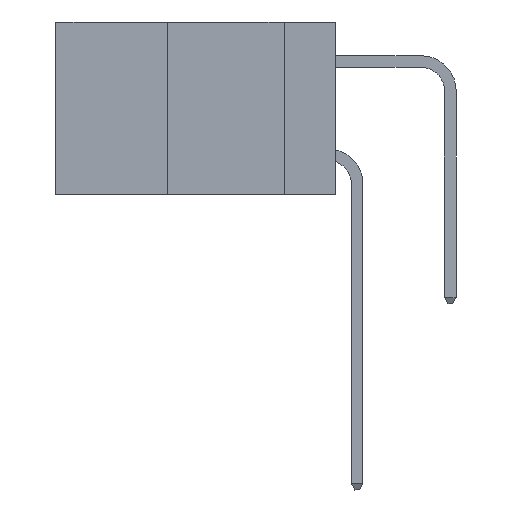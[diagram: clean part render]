
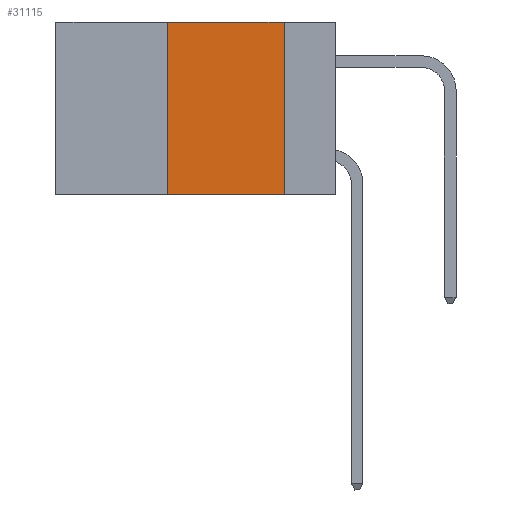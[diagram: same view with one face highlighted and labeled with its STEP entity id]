
A CAD part, left-side view. The second image highlights one B-rep face of the part: STEP entity #31115.
In plain terms, the highlighted planar face has unit normal (-1, 0, 0).
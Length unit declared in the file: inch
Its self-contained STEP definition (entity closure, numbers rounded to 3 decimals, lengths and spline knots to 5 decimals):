
#439 = VERTEX_POINT ( 'NONE', #29322 ) ;
#998 = EDGE_CURVE ( 'NONE', #26882, #2887, #19389, .T. ) ;
#1712 = CARTESIAN_POINT ( 'NONE',  ( 0., 0.36, 0. ) ) ;
#2887 = VERTEX_POINT ( 'NONE', #19974 ) ;
#2962 = AXIS2_PLACEMENT_3D ( 'NONE', #10636, #27535, #10545 ) ;
#3254 = CARTESIAN_POINT ( 'NONE',  ( 0., 0.6, -0.37 ) ) ;
#6092 = CARTESIAN_POINT ( 'NONE',  ( 0., 0.11, 0. ) ) ;
#8048 = VECTOR ( 'NONE', #12222, 39.37008 ) ;
#9205 = EDGE_CURVE ( 'NONE', #2887, #439, #23716, .T. ) ;
#10545 = DIRECTION ( 'NONE',  ( 0., 0., -1. ) ) ;
#10636 = CARTESIAN_POINT ( 'NONE',  ( 0., 0.6, 0. ) ) ;
#11877 = EDGE_LOOP ( 'NONE', ( #29305, #13798, #22561, #20079 ) ) ;
#12222 = DIRECTION ( 'NONE',  ( 0., -1., 0. ) ) ;
#13063 = LINE ( 'NONE', #1712, #20630 ) ;
#13798 = ORIENTED_EDGE ( 'NONE', *, *, #998, .F. ) ;
#14108 = CARTESIAN_POINT ( 'NONE',  ( 0., 0.36, -0.37 ) ) ;
#14882 = EDGE_CURVE ( 'NONE', #16579, #26882, #13063, .T. ) ;
#16579 = VERTEX_POINT ( 'NONE', #14108 ) ;
#17834 = PLANE ( 'NONE',  #2962 ) ;
#18249 = DIRECTION ( 'NONE',  ( 0., 0., -1. ) ) ;
#19389 = LINE ( 'NONE', #21782, #8048 ) ;
#19974 = CARTESIAN_POINT ( 'NONE',  ( 0., 0.11, 0. ) ) ;
#20079 = ORIENTED_EDGE ( 'NONE', *, *, #21884, .T. ) ;
#20208 = DIRECTION ( 'NONE',  ( 0., -1., 0. ) ) ;
#20630 = VECTOR ( 'NONE', #30714, 39.37008 ) ;
#21782 = CARTESIAN_POINT ( 'NONE',  ( 0., 0.6, 0. ) ) ;
#21884 = EDGE_CURVE ( 'NONE', #16579, #439, #30932, .T. ) ;
#22561 = ORIENTED_EDGE ( 'NONE', *, *, #14882, .F. ) ;
#23716 = LINE ( 'NONE', #6092, #28235 ) ;
#26882 = VERTEX_POINT ( 'NONE', #28837 ) ;
#27535 = DIRECTION ( 'NONE',  ( 1., 0., 0. ) ) ;
#28235 = VECTOR ( 'NONE', #18249, 39.37008 ) ;
#28837 = CARTESIAN_POINT ( 'NONE',  ( 0., 0.36, 0. ) ) ;
#29176 = FACE_OUTER_BOUND ( 'NONE', #11877, .T. ) ;
#29305 = ORIENTED_EDGE ( 'NONE', *, *, #9205, .F. ) ;
#29322 = CARTESIAN_POINT ( 'NONE',  ( 0., 0.11, -0.37 ) ) ;
#30714 = DIRECTION ( 'NONE',  ( 0., 0., 1. ) ) ;
#30932 = LINE ( 'NONE', #3254, #31308 ) ;
#31115 = ADVANCED_FACE ( 'NONE', ( #29176 ), #17834, .F. ) ;
#31308 = VECTOR ( 'NONE', #20208, 39.37008 ) ;
